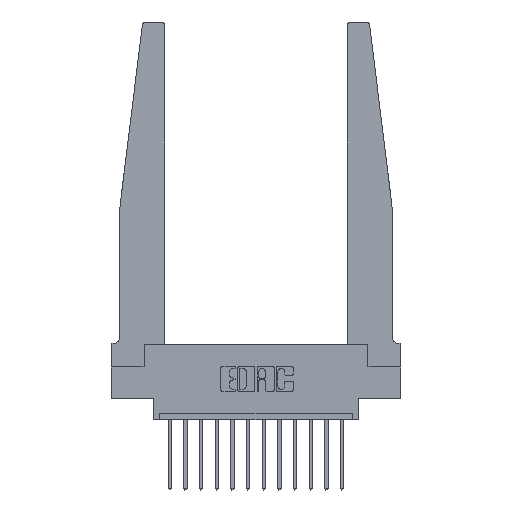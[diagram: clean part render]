
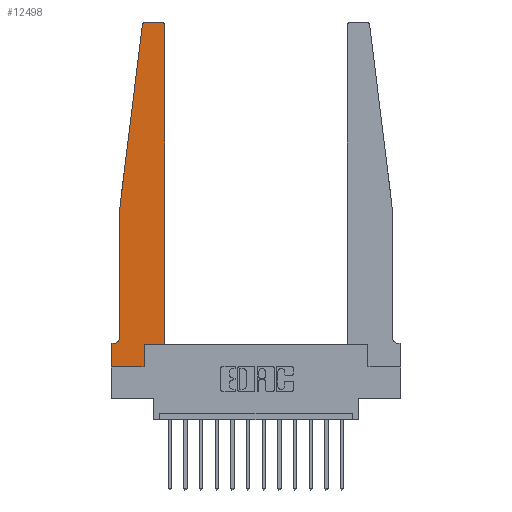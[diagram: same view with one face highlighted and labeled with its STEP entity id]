
A CAD part, top view. The second image highlights one B-rep face of the part: STEP entity #12498.
In plain terms, the highlighted planar face has unit normal (0, 0, 1).
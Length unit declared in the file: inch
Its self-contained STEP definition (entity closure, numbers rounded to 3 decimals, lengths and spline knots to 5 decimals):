
#231 = ORIENTED_EDGE ( 'NONE', *, *, #1318, .T. ) ;
#350 = DIRECTION ( 'NONE',  ( -1., 0., 0. ) ) ;
#399 = ORIENTED_EDGE ( 'NONE', *, *, #9240, .T. ) ;
#488 = ORIENTED_EDGE ( 'NONE', *, *, #14028, .T. ) ;
#559 = EDGE_LOOP ( 'NONE', ( #2904, #7471, #805, #399, #8568, #4506, #231, #8555, #4317, #488, #1365, #16438 ) ) ;
#805 = ORIENTED_EDGE ( 'NONE', *, *, #1628, .T. ) ;
#1258 = LINE ( 'NONE', #6508, #3453 ) ;
#1318 = EDGE_CURVE ( 'NONE', #4289, #13770, #6383, .T. ) ;
#1365 = ORIENTED_EDGE ( 'NONE', *, *, #1795, .T. ) ;
#1416 = DIRECTION ( 'NONE',  ( 1., 0., 0. ) ) ;
#1628 = EDGE_CURVE ( 'NONE', #2844, #16328, #11522, .T. ) ;
#1745 = DIRECTION ( 'NONE',  ( -1., 0., 0. ) ) ;
#1795 = EDGE_CURVE ( 'NONE', #7514, #7448, #6685, .T. ) ;
#1804 = CARTESIAN_POINT ( 'NONE',  ( 0.395, 2.72, 0.37 ) ) ;
#1851 = CARTESIAN_POINT ( 'NONE',  ( 0.065, 1.25, 0.37 ) ) ;
#1874 = DIRECTION ( 'NONE',  ( 0., 0., 1. ) ) ;
#1909 = VECTOR ( 'NONE', #10173, 39.37008 ) ;
#2187 = EDGE_CURVE ( 'NONE', #5755, #4289, #3852, .T. ) ;
#2623 = CARTESIAN_POINT ( 'NONE',  ( 0.425, 2.72, 0.37 ) ) ;
#2767 = CARTESIAN_POINT ( 'NONE',  ( 0.425, 0.18, 0.37 ) ) ;
#2798 = CIRCLE ( 'NONE', #3618, 0.03 ) ;
#2844 = VERTEX_POINT ( 'NONE', #10434 ) ;
#2860 = LINE ( 'NONE', #15572, #11517 ) ;
#2904 = ORIENTED_EDGE ( 'NONE', *, *, #13480, .T. ) ;
#3198 = DIRECTION ( 'NONE',  ( 0., -1., 0. ) ) ;
#3320 = DIRECTION ( 'NONE',  ( 0., 0., 1. ) ) ;
#3431 = AXIS2_PLACEMENT_3D ( 'NONE', #9910, #1874, #14835 ) ;
#3442 = VECTOR ( 'NONE', #350, 39.37008 ) ;
#3453 = VECTOR ( 'NONE', #1416, 39.37008 ) ;
#3618 = AXIS2_PLACEMENT_3D ( 'NONE', #9363, #9453, #15567 ) ;
#3642 = CIRCLE ( 'NONE', #10489, 0.05 ) ;
#3651 = CARTESIAN_POINT ( 'NONE',  ( 0., 0.1875, 0.37 ) ) ;
#3852 = LINE ( 'NONE', #14351, #16047 ) ;
#3971 = CARTESIAN_POINT ( 'NONE',  ( 0.065, 0.2375, 0.37 ) ) ;
#4091 = VERTEX_POINT ( 'NONE', #11893 ) ;
#4289 = VERTEX_POINT ( 'NONE', #3651 ) ;
#4317 = ORIENTED_EDGE ( 'NONE', *, *, #5988, .T. ) ;
#4506 = ORIENTED_EDGE ( 'NONE', *, *, #2187, .T. ) ;
#4879 = VERTEX_POINT ( 'NONE', #3971 ) ;
#4956 = DIRECTION ( 'NONE',  ( 1., 0., 0. ) ) ;
#4990 = DIRECTION ( 'NONE',  ( -0.122, -0.992, 0. ) ) ;
#5755 = VERTEX_POINT ( 'NONE', #16695 ) ;
#5988 = EDGE_CURVE ( 'NONE', #6663, #4091, #2860, .T. ) ;
#6383 = LINE ( 'NONE', #10342, #1909 ) ;
#6508 = CARTESIAN_POINT ( 'NONE',  ( 0.425, 0.18, 0.37 ) ) ;
#6567 = CARTESIAN_POINT ( 'NONE',  ( 0., 0., 0.37 ) ) ;
#6663 = VERTEX_POINT ( 'NONE', #8065 ) ;
#6685 = LINE ( 'NONE', #2767, #9836 ) ;
#6720 = LINE ( 'NONE', #12132, #3442 ) ;
#7448 = VERTEX_POINT ( 'NONE', #2623 ) ;
#7471 = ORIENTED_EDGE ( 'NONE', *, *, #7780, .T. ) ;
#7514 = VERTEX_POINT ( 'NONE', #13466 ) ;
#7515 = VECTOR ( 'NONE', #4956, 39.37008 ) ;
#7780 = EDGE_CURVE ( 'NONE', #12671, #2844, #2798, .T. ) ;
#7926 = DIRECTION ( 'NONE',  ( 0., 1., 0. ) ) ;
#8065 = CARTESIAN_POINT ( 'NONE',  ( 0.2605, 0., 0.37 ) ) ;
#8555 = ORIENTED_EDGE ( 'NONE', *, *, #11699, .T. ) ;
#8568 = ORIENTED_EDGE ( 'NONE', *, *, #10291, .T. ) ;
#8569 = DIRECTION ( 'NONE',  ( 1., 0., 0. ) ) ;
#9106 = DIRECTION ( 'NONE',  ( 0., 1., 0. ) ) ;
#9240 = EDGE_CURVE ( 'NONE', #16328, #4879, #14893, .T. ) ;
#9363 = CARTESIAN_POINT ( 'NONE',  ( 0.27653, 2.72, 0.37 ) ) ;
#9434 = CARTESIAN_POINT ( 'NONE',  ( 0.015, 0.2375, 0.37 ) ) ;
#9453 = DIRECTION ( 'NONE',  ( 0., 0., 1. ) ) ;
#9636 = CARTESIAN_POINT ( 'NONE',  ( 0.27653, 2.75, 0.37 ) ) ;
#9836 = VECTOR ( 'NONE', #9106, 39.37008 ) ;
#9910 = CARTESIAN_POINT ( 'NONE',  ( 0., 0.1875, 0.37 ) ) ;
#10173 = DIRECTION ( 'NONE',  ( 0., -1., 0. ) ) ;
#10291 = EDGE_CURVE ( 'NONE', #4879, #5755, #3642, .T. ) ;
#10338 = AXIS2_PLACEMENT_3D ( 'NONE', #1804, #3320, #8569 ) ;
#10342 = CARTESIAN_POINT ( 'NONE',  ( 0., 0., 0.37 ) ) ;
#10434 = CARTESIAN_POINT ( 'NONE',  ( 0.24675, 2.72367, 0.37 ) ) ;
#10489 = AXIS2_PLACEMENT_3D ( 'NONE', #9434, #16061, #1745 ) ;
#11287 = CARTESIAN_POINT ( 'NONE',  ( 0., 0., 0.37 ) ) ;
#11517 = VECTOR ( 'NONE', #7926, 39.37008 ) ;
#11522 = LINE ( 'NONE', #13879, #13092 ) ;
#11621 = CARTESIAN_POINT ( 'NONE',  ( 0.065, 1.25, 0.37 ) ) ;
#11699 = EDGE_CURVE ( 'NONE', #13770, #6663, #15452, .T. ) ;
#11893 = CARTESIAN_POINT ( 'NONE',  ( 0.2605, 0.18, 0.37 ) ) ;
#11941 = CARTESIAN_POINT ( 'NONE',  ( 0.395, 2.75, 0.37 ) ) ;
#12132 = CARTESIAN_POINT ( 'NONE',  ( 0.25, 2.75, 0.37 ) ) ;
#12302 = FACE_OUTER_BOUND ( 'NONE', #559, .T. ) ;
#12498 = ADVANCED_FACE ( 'NONE', ( #12302 ), #16196, .T. ) ;
#12671 = VERTEX_POINT ( 'NONE', #9636 ) ;
#13055 = CIRCLE ( 'NONE', #10338, 0.03 ) ;
#13092 = VECTOR ( 'NONE', #4990, 39.37008 ) ;
#13211 = VECTOR ( 'NONE', #3198, 39.37008 ) ;
#13466 = CARTESIAN_POINT ( 'NONE',  ( 0.425, 0.18, 0.37 ) ) ;
#13480 = EDGE_CURVE ( 'NONE', #13957, #12671, #6720, .T. ) ;
#13770 = VERTEX_POINT ( 'NONE', #11287 ) ;
#13879 = CARTESIAN_POINT ( 'NONE',  ( 0.065, 1.25, 0.37 ) ) ;
#13957 = VERTEX_POINT ( 'NONE', #11941 ) ;
#14028 = EDGE_CURVE ( 'NONE', #4091, #7514, #1258, .T. ) ;
#14351 = CARTESIAN_POINT ( 'NONE',  ( 0.065, 0.1875, 0.37 ) ) ;
#14835 = DIRECTION ( 'NONE',  ( 1., 0., 0. ) ) ;
#14893 = LINE ( 'NONE', #1851, #13211 ) ;
#15452 = LINE ( 'NONE', #6567, #7515 ) ;
#15546 = DIRECTION ( 'NONE',  ( -1., 0., 0. ) ) ;
#15567 = DIRECTION ( 'NONE',  ( 1., 0., 0. ) ) ;
#15572 = CARTESIAN_POINT ( 'NONE',  ( 0.2605, 0.18, 0.37 ) ) ;
#16046 = EDGE_CURVE ( 'NONE', #7448, #13957, #13055, .T. ) ;
#16047 = VECTOR ( 'NONE', #15546, 39.37008 ) ;
#16061 = DIRECTION ( 'NONE',  ( 0., 0., -1. ) ) ;
#16196 = PLANE ( 'NONE',  #3431 ) ;
#16328 = VERTEX_POINT ( 'NONE', #11621 ) ;
#16438 = ORIENTED_EDGE ( 'NONE', *, *, #16046, .T. ) ;
#16695 = CARTESIAN_POINT ( 'NONE',  ( 0.015, 0.1875, 0.37 ) ) ;
